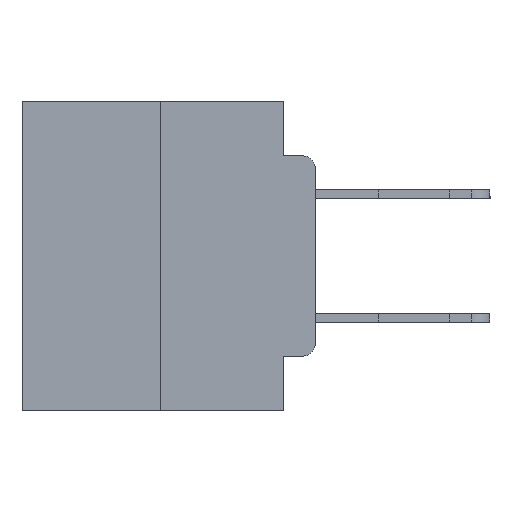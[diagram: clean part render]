
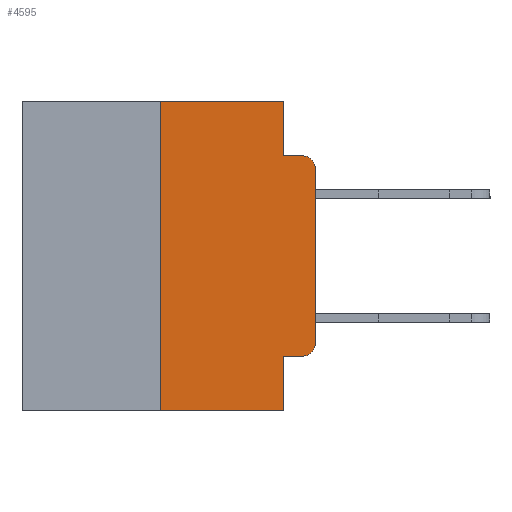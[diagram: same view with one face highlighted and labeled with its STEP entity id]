
A CAD part, left-side view. The second image highlights one B-rep face of the part: STEP entity #4595.
In plain terms, the highlighted planar face has unit normal (-1, 0, 0).
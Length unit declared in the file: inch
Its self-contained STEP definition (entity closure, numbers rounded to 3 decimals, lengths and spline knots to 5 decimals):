
#355 = CARTESIAN_POINT ( 'NONE',  ( 0., 0.051, 0. ) ) ;
#615 = EDGE_CURVE ( 'NONE', #14025, #6242, #25003, .T. ) ;
#1012 = DIRECTION ( 'NONE',  ( 0., 0., -1. ) ) ;
#1407 = FACE_OUTER_BOUND ( 'NONE', #21728, .T. ) ;
#1514 = EDGE_CURVE ( 'NONE', #22903, #14025, #13387, .T. ) ;
#1641 = DIRECTION ( 'NONE',  ( 1., 0., 0. ) ) ;
#1669 = EDGE_CURVE ( 'NONE', #6987, #10780, #14953, .T. ) ;
#1685 = LINE ( 'NONE', #14981, #16617 ) ;
#2066 = ORIENTED_EDGE ( 'NONE', *, *, #7503, .F. ) ;
#2413 = CARTESIAN_POINT ( 'NONE',  ( 0., 0.25, 0. ) ) ;
#3413 = LINE ( 'NONE', #17834, #13604 ) ;
#3426 = CARTESIAN_POINT ( 'NONE',  ( 0., 0.051, -0.4115 ) ) ;
#3560 = EDGE_CURVE ( 'NONE', #12065, #10780, #3413, .T. ) ;
#4421 = DIRECTION ( 'NONE',  ( 0., 0., -1. ) ) ;
#4595 = ADVANCED_FACE ( 'NONE', ( #1407 ), #24397, .F. ) ;
#4856 = EDGE_CURVE ( 'NONE', #9471, #24818, #17995, .T. ) ;
#4915 = LINE ( 'NONE', #3426, #9661 ) ;
#5655 = CIRCLE ( 'NONE', #13174, 0.02 ) ;
#6201 = EDGE_CURVE ( 'NONE', #24818, #17525, #18522, .T. ) ;
#6242 = VERTEX_POINT ( 'NONE', #16717 ) ;
#6602 = DIRECTION ( 'NONE',  ( 0., 0., 1. ) ) ;
#6987 = VERTEX_POINT ( 'NONE', #7231 ) ;
#7231 = CARTESIAN_POINT ( 'NONE',  ( 0., 0.25, -0.5 ) ) ;
#7292 = VECTOR ( 'NONE', #7758, 39.37008 ) ;
#7308 = CARTESIAN_POINT ( 'NONE',  ( 0., 0.02, -0.4115 ) ) ;
#7503 = EDGE_CURVE ( 'NONE', #17525, #13957, #1685, .T. ) ;
#7716 = CARTESIAN_POINT ( 'NONE',  ( 0., 0., -0.3915 ) ) ;
#7758 = DIRECTION ( 'NONE',  ( 0., -1., 0. ) ) ;
#7990 = VECTOR ( 'NONE', #22568, 39.37008 ) ;
#8016 = CARTESIAN_POINT ( 'NONE',  ( 0., 0.051, 0. ) ) ;
#8441 = ORIENTED_EDGE ( 'NONE', *, *, #4856, .F. ) ;
#8951 = VECTOR ( 'NONE', #6602, 39.37008 ) ;
#9038 = DIRECTION ( 'NONE',  ( 0., -1., 0. ) ) ;
#9276 = CARTESIAN_POINT ( 'NONE',  ( 0., 0.051, -0.4115 ) ) ;
#9471 = VERTEX_POINT ( 'NONE', #16481 ) ;
#9661 = VECTOR ( 'NONE', #21615, 39.37008 ) ;
#10780 = VERTEX_POINT ( 'NONE', #20759 ) ;
#11776 = CARTESIAN_POINT ( 'NONE',  ( 0., 0.473, 0. ) ) ;
#12065 = VERTEX_POINT ( 'NONE', #9276 ) ;
#12129 = DIRECTION ( 'NONE',  ( 0., 0., -1. ) ) ;
#13174 = AXIS2_PLACEMENT_3D ( 'NONE', #25236, #13221, #1012 ) ;
#13221 = DIRECTION ( 'NONE',  ( -1., 0., 0. ) ) ;
#13387 = CIRCLE ( 'NONE', #15007, 0.02 ) ;
#13604 = VECTOR ( 'NONE', #18854, 39.37008 ) ;
#13699 = CARTESIAN_POINT ( 'NONE',  ( 0., 0.473, 0. ) ) ;
#13710 = DIRECTION ( 'NONE',  ( -1., 0., 0. ) ) ;
#13957 = VERTEX_POINT ( 'NONE', #25640 ) ;
#14025 = VERTEX_POINT ( 'NONE', #7716 ) ;
#14337 = VECTOR ( 'NONE', #19502, 39.37008 ) ;
#14953 = LINE ( 'NONE', #21601, #14337 ) ;
#14981 = CARTESIAN_POINT ( 'NONE',  ( 0., 0.051, -0.0885 ) ) ;
#15007 = AXIS2_PLACEMENT_3D ( 'NONE', #23712, #13710, #12129 ) ;
#15036 = ORIENTED_EDGE ( 'NONE', *, *, #615, .T. ) ;
#15082 = ORIENTED_EDGE ( 'NONE', *, *, #1669, .T. ) ;
#15615 = CARTESIAN_POINT ( 'NONE',  ( 0., 0., 0. ) ) ;
#16364 = ORIENTED_EDGE ( 'NONE', *, *, #24561, .T. ) ;
#16481 = CARTESIAN_POINT ( 'NONE',  ( 0., 0.25, 0. ) ) ;
#16617 = VECTOR ( 'NONE', #9038, 39.37008 ) ;
#16672 = ORIENTED_EDGE ( 'NONE', *, *, #1514, .T. ) ;
#16717 = CARTESIAN_POINT ( 'NONE',  ( 0., 0., -0.1085 ) ) ;
#17294 = VECTOR ( 'NONE', #4421, 39.37008 ) ;
#17525 = VERTEX_POINT ( 'NONE', #20984 ) ;
#17574 = ORIENTED_EDGE ( 'NONE', *, *, #18055, .F. ) ;
#17834 = CARTESIAN_POINT ( 'NONE',  ( 0., 0.051, 0. ) ) ;
#17995 = LINE ( 'NONE', #11776, #7292 ) ;
#18055 = EDGE_CURVE ( 'NONE', #6987, #9471, #18643, .T. ) ;
#18481 = ORIENTED_EDGE ( 'NONE', *, *, #6201, .F. ) ;
#18522 = LINE ( 'NONE', #355, #17294 ) ;
#18643 = LINE ( 'NONE', #2413, #7990 ) ;
#18779 = ORIENTED_EDGE ( 'NONE', *, *, #25912, .T. ) ;
#18854 = DIRECTION ( 'NONE',  ( 0., 0., -1. ) ) ;
#19502 = DIRECTION ( 'NONE',  ( 0., -1., 0. ) ) ;
#20759 = CARTESIAN_POINT ( 'NONE',  ( 0., 0.051, -0.5 ) ) ;
#20984 = CARTESIAN_POINT ( 'NONE',  ( 0., 0.051, -0.0885 ) ) ;
#21601 = CARTESIAN_POINT ( 'NONE',  ( 0., 0.473, -0.5 ) ) ;
#21615 = DIRECTION ( 'NONE',  ( 0., -1., 0. ) ) ;
#21728 = EDGE_LOOP ( 'NONE', ( #15036, #16364, #2066, #18481, #8441, #17574, #15082, #25735, #18779, #16672 ) ) ;
#22116 = AXIS2_PLACEMENT_3D ( 'NONE', #13699, #1641, #25862 ) ;
#22568 = DIRECTION ( 'NONE',  ( 0., 0., 1. ) ) ;
#22903 = VERTEX_POINT ( 'NONE', #7308 ) ;
#23712 = CARTESIAN_POINT ( 'NONE',  ( 0., 0.02, -0.3915 ) ) ;
#24397 = PLANE ( 'NONE',  #22116 ) ;
#24561 = EDGE_CURVE ( 'NONE', #6242, #13957, #5655, .T. ) ;
#24818 = VERTEX_POINT ( 'NONE', #8016 ) ;
#25003 = LINE ( 'NONE', #15615, #8951 ) ;
#25236 = CARTESIAN_POINT ( 'NONE',  ( 0., 0.02, -0.1085 ) ) ;
#25640 = CARTESIAN_POINT ( 'NONE',  ( 0., 0.02, -0.0885 ) ) ;
#25735 = ORIENTED_EDGE ( 'NONE', *, *, #3560, .F. ) ;
#25862 = DIRECTION ( 'NONE',  ( 0., 0., -1. ) ) ;
#25912 = EDGE_CURVE ( 'NONE', #12065, #22903, #4915, .T. ) ;
